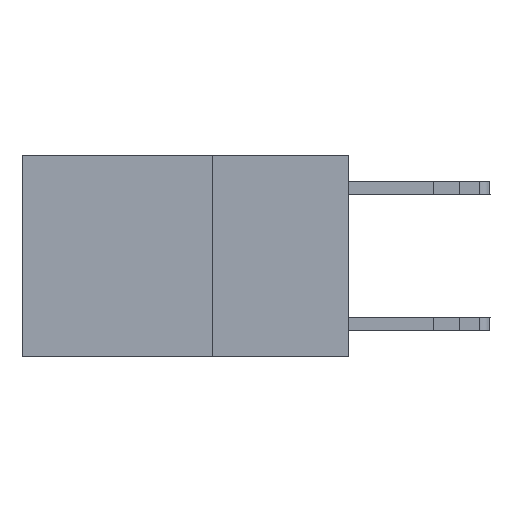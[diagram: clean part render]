
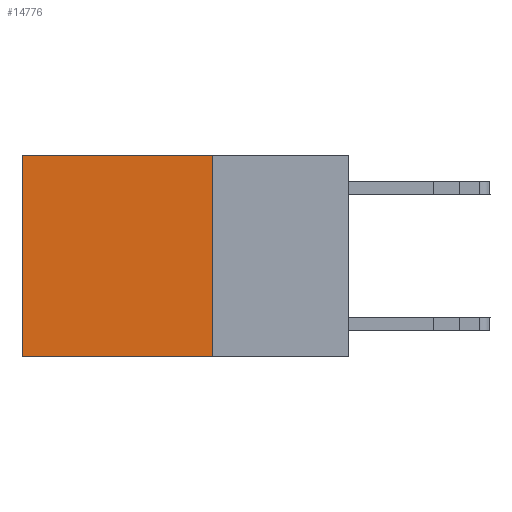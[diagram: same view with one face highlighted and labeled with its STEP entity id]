
A CAD part, left-side view. The second image highlights one B-rep face of the part: STEP entity #14776.
In plain terms, the highlighted planar face has unit normal (-1, 0, 0).
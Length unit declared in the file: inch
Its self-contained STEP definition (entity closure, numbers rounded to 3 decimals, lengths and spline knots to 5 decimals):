
#392 = CARTESIAN_POINT ( 'NONE',  ( 0.2625, 0.25, -0.37 ) ) ;
#485 = EDGE_LOOP ( 'NONE', ( #18046, #18145, #3264, #1175 ) ) ;
#1175 = ORIENTED_EDGE ( 'NONE', *, *, #1932, .T. ) ;
#1207 = DIRECTION ( 'NONE',  ( 1., 0., 0. ) ) ;
#1260 = LINE ( 'NONE', #7431, #12507 ) ;
#1789 = AXIS2_PLACEMENT_3D ( 'NONE', #19754, #1207, #10526 ) ;
#1902 = CARTESIAN_POINT ( 'NONE',  ( 0.2625, 0.25, 0. ) ) ;
#1932 = EDGE_CURVE ( 'NONE', #9643, #8806, #13432, .T. ) ;
#2124 = VECTOR ( 'NONE', #12701, 39.37008 ) ;
#2524 = PLANE ( 'NONE',  #1789 ) ;
#3264 = ORIENTED_EDGE ( 'NONE', *, *, #7898, .F. ) ;
#3648 = VERTEX_POINT ( 'NONE', #11386 ) ;
#4724 = VERTEX_POINT ( 'NONE', #11187 ) ;
#5660 = DIRECTION ( 'NONE',  ( 0., 0., -1. ) ) ;
#6867 = VECTOR ( 'NONE', #16081, 39.37008 ) ;
#7431 = CARTESIAN_POINT ( 'NONE',  ( 0.2625, 0.6, 0. ) ) ;
#7898 = EDGE_CURVE ( 'NONE', #9643, #4724, #19274, .T. ) ;
#8642 = CARTESIAN_POINT ( 'NONE',  ( 0.2625, 0.25, 0. ) ) ;
#8806 = VERTEX_POINT ( 'NONE', #17608 ) ;
#9600 = EDGE_CURVE ( 'NONE', #4724, #3648, #9802, .T. ) ;
#9643 = VERTEX_POINT ( 'NONE', #1902 ) ;
#9802 = LINE ( 'NONE', #392, #6867 ) ;
#10219 = FACE_OUTER_BOUND ( 'NONE', #485, .T. ) ;
#10526 = DIRECTION ( 'NONE',  ( 0., 0., -1. ) ) ;
#10999 = VECTOR ( 'NONE', #5660, 39.37008 ) ;
#11187 = CARTESIAN_POINT ( 'NONE',  ( 0.2625, 0.25, -0.37 ) ) ;
#11386 = CARTESIAN_POINT ( 'NONE',  ( 0.2625, 0.6, -0.37 ) ) ;
#12507 = VECTOR ( 'NONE', #17897, 39.37008 ) ;
#12701 = DIRECTION ( 'NONE',  ( 0., 1., 0. ) ) ;
#13432 = LINE ( 'NONE', #15731, #2124 ) ;
#14776 = ADVANCED_FACE ( 'NONE', ( #10219 ), #2524, .F. ) ;
#15731 = CARTESIAN_POINT ( 'NONE',  ( 0.2625, 0.25, 0. ) ) ;
#16081 = DIRECTION ( 'NONE',  ( 0., 1., 0. ) ) ;
#17182 = EDGE_CURVE ( 'NONE', #8806, #3648, #1260, .T. ) ;
#17608 = CARTESIAN_POINT ( 'NONE',  ( 0.2625, 0.6, 0. ) ) ;
#17897 = DIRECTION ( 'NONE',  ( 0., 0., -1. ) ) ;
#18046 = ORIENTED_EDGE ( 'NONE', *, *, #17182, .T. ) ;
#18145 = ORIENTED_EDGE ( 'NONE', *, *, #9600, .F. ) ;
#19274 = LINE ( 'NONE', #8642, #10999 ) ;
#19754 = CARTESIAN_POINT ( 'NONE',  ( 0.2625, 0.25, 0. ) ) ;
